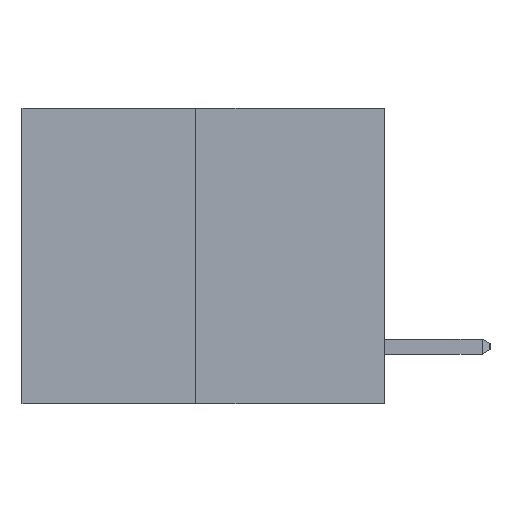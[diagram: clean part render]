
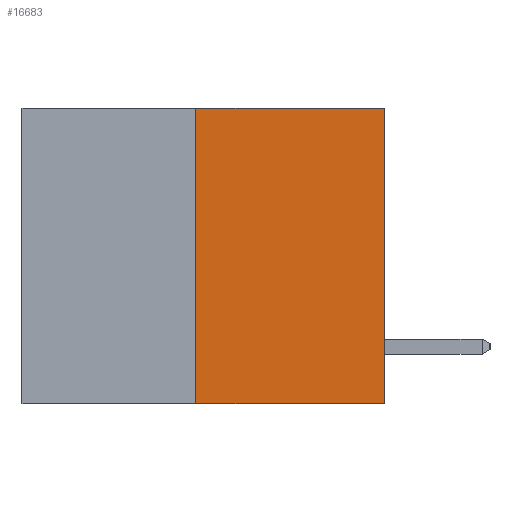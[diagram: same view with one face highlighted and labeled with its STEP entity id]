
A CAD part, left-side view. The second image highlights one B-rep face of the part: STEP entity #16683.
In plain terms, the highlighted planar face has unit normal (-1, 0, 0).
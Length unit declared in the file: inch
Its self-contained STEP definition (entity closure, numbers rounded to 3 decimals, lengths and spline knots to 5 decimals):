
#1976 = ORIENTED_EDGE ( 'NONE', *, *, #19455, .F. ) ;
#2329 = VECTOR ( 'NONE', #8672, 39.37008 ) ;
#2409 = DIRECTION ( 'NONE',  ( 0., 0., -1. ) ) ;
#2630 = CARTESIAN_POINT ( 'NONE',  ( 0., 0.6, 0. ) ) ;
#2933 = VERTEX_POINT ( 'NONE', #5431 ) ;
#3011 = VERTEX_POINT ( 'NONE', #17189 ) ;
#3347 = VERTEX_POINT ( 'NONE', #9925 ) ;
#3798 = CARTESIAN_POINT ( 'NONE',  ( 0., 0.312, -0.49 ) ) ;
#5431 = CARTESIAN_POINT ( 'NONE',  ( 0., 0., 0. ) ) ;
#5546 = AXIS2_PLACEMENT_3D ( 'NONE', #2630, #18769, #2409 ) ;
#6179 = CARTESIAN_POINT ( 'NONE',  ( 0., 0.312, -0.49 ) ) ;
#6960 = FACE_OUTER_BOUND ( 'NONE', #9029, .T. ) ;
#7949 = DIRECTION ( 'NONE',  ( 0., 0., 1. ) ) ;
#8672 = DIRECTION ( 'NONE',  ( 0., 0., 1. ) ) ;
#9029 = EDGE_LOOP ( 'NONE', ( #18596, #19062, #15203, #1976 ) ) ;
#9157 = EDGE_CURVE ( 'NONE', #15079, #3011, #10216, .T. ) ;
#9925 = CARTESIAN_POINT ( 'NONE',  ( 0., 0., -0.49 ) ) ;
#9973 = CARTESIAN_POINT ( 'NONE',  ( 0., 0., 0. ) ) ;
#10216 = LINE ( 'NONE', #3798, #2329 ) ;
#10430 = LINE ( 'NONE', #18848, #19157 ) ;
#12559 = CARTESIAN_POINT ( 'NONE',  ( 0., 0.6, -0.49 ) ) ;
#13831 = EDGE_CURVE ( 'NONE', #15079, #3347, #20707, .T. ) ;
#15079 = VERTEX_POINT ( 'NONE', #6179 ) ;
#15203 = ORIENTED_EDGE ( 'NONE', *, *, #20924, .T. ) ;
#15249 = LINE ( 'NONE', #9973, #20888 ) ;
#16683 = ADVANCED_FACE ( 'NONE', ( #6960 ), #18700, .F. ) ;
#17102 = VECTOR ( 'NONE', #19155, 39.37008 ) ;
#17189 = CARTESIAN_POINT ( 'NONE',  ( 0., 0.312, 0. ) ) ;
#18596 = ORIENTED_EDGE ( 'NONE', *, *, #9157, .F. ) ;
#18700 = PLANE ( 'NONE',  #5546 ) ;
#18769 = DIRECTION ( 'NONE',  ( 1., 0., 0. ) ) ;
#18848 = CARTESIAN_POINT ( 'NONE',  ( 0., 0.6, 0. ) ) ;
#18991 = DIRECTION ( 'NONE',  ( 0., -1., 0. ) ) ;
#19062 = ORIENTED_EDGE ( 'NONE', *, *, #13831, .T. ) ;
#19155 = DIRECTION ( 'NONE',  ( 0., -1., 0. ) ) ;
#19157 = VECTOR ( 'NONE', #18991, 39.37008 ) ;
#19455 = EDGE_CURVE ( 'NONE', #3011, #2933, #10430, .T. ) ;
#20707 = LINE ( 'NONE', #12559, #17102 ) ;
#20888 = VECTOR ( 'NONE', #7949, 39.37008 ) ;
#20924 = EDGE_CURVE ( 'NONE', #3347, #2933, #15249, .T. ) ;
